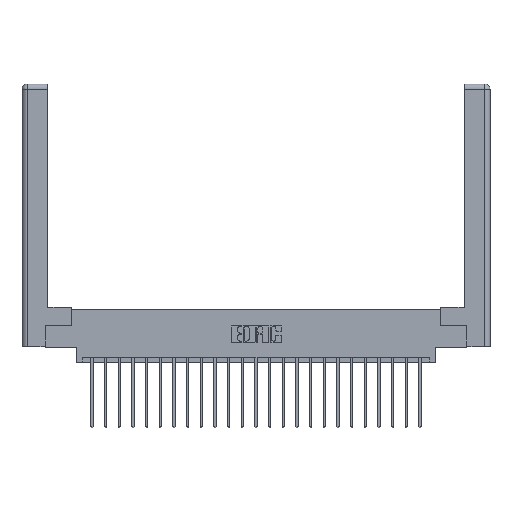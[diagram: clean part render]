
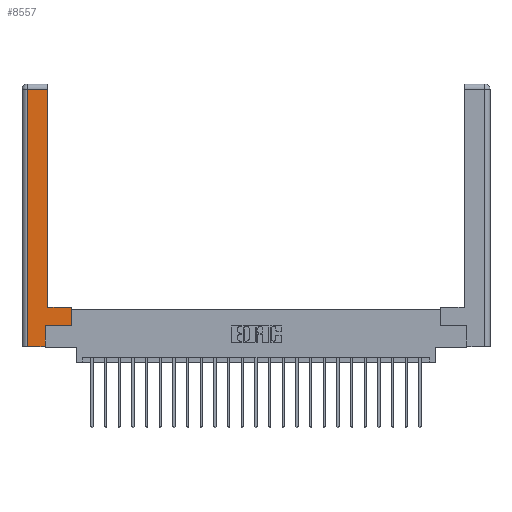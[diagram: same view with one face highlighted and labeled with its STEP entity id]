
A CAD part, top view. The second image highlights one B-rep face of the part: STEP entity #8557.
In plain terms, the highlighted planar face has unit normal (0, 0, 1).
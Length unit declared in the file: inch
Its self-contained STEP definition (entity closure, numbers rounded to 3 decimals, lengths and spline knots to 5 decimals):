
#236 = VERTEX_POINT ( 'NONE', #16291 ) ;
#309 = DIRECTION ( 'NONE',  ( -1., 0., 0. ) ) ;
#493 = LINE ( 'NONE', #4490, #4329 ) ;
#516 = CARTESIAN_POINT ( 'NONE',  ( 0.295, 2.94, 0. ) ) ;
#560 = VERTEX_POINT ( 'NONE', #11303 ) ;
#584 = LINE ( 'NONE', #3788, #7951 ) ;
#1024 = ORIENTED_EDGE ( 'NONE', *, *, #7927, .T. ) ;
#1229 = EDGE_CURVE ( 'NONE', #236, #560, #584, .T. ) ;
#1248 = EDGE_CURVE ( 'NONE', #13226, #10148, #17660, .T. ) ;
#2420 = CARTESIAN_POINT ( 'NONE',  ( 0.295, 3., 0. ) ) ;
#3190 = CARTESIAN_POINT ( 'NONE',  ( 0.295, 0.45, 0. ) ) ;
#3208 = DIRECTION ( 'NONE',  ( 0., 1., 0. ) ) ;
#3457 = EDGE_CURVE ( 'NONE', #4416, #13226, #493, .T. ) ;
#3673 = EDGE_CURVE ( 'NONE', #13757, #4416, #9888, .T. ) ;
#3763 = CARTESIAN_POINT ( 'NONE',  ( 0.265, 0., 0. ) ) ;
#3788 = CARTESIAN_POINT ( 'NONE',  ( 0.565, 0.245, 0. ) ) ;
#4329 = VECTOR ( 'NONE', #8517, 39.37008 ) ;
#4416 = VERTEX_POINT ( 'NONE', #516 ) ;
#4490 = CARTESIAN_POINT ( 'NONE',  ( 0.0615, 2.94, 0. ) ) ;
#5442 = CARTESIAN_POINT ( 'NONE',  ( 0.0615, 0., 0. ) ) ;
#6892 = DIRECTION ( 'NONE',  ( 0., 0., -1. ) ) ;
#6925 = CARTESIAN_POINT ( 'NONE',  ( 0.265, 0.245, 0. ) ) ;
#7927 = EDGE_CURVE ( 'NONE', #560, #14397, #12509, .T. ) ;
#7951 = VECTOR ( 'NONE', #22508, 39.37008 ) ;
#8245 = EDGE_CURVE ( 'NONE', #13904, #236, #17812, .T. ) ;
#8517 = DIRECTION ( 'NONE',  ( -1., 0., 0. ) ) ;
#8557 = ADVANCED_FACE ( 'NONE', ( #15566 ), #8765, .F. ) ;
#8765 = PLANE ( 'NONE',  #18455 ) ;
#9130 = ORIENTED_EDGE ( 'NONE', *, *, #23506, .T. ) ;
#9276 = VECTOR ( 'NONE', #3208, 39.37008 ) ;
#9432 = ORIENTED_EDGE ( 'NONE', *, *, #8245, .T. ) ;
#9701 = CARTESIAN_POINT ( 'NONE',  ( 0.0615, 0., 0. ) ) ;
#9888 = LINE ( 'NONE', #2420, #10201 ) ;
#10148 = VERTEX_POINT ( 'NONE', #9701 ) ;
#10201 = VECTOR ( 'NONE', #21325, 39.37008 ) ;
#10463 = VECTOR ( 'NONE', #16223, 39.37008 ) ;
#10732 = EDGE_LOOP ( 'NONE', ( #18610, #23179, #24391, #9130, #9432, #20119, #1024, #12828 ) ) ;
#11079 = CARTESIAN_POINT ( 'NONE',  ( 0.295, 0.45, 0. ) ) ;
#11303 = CARTESIAN_POINT ( 'NONE',  ( 0.565, 0.245, 0. ) ) ;
#12509 = LINE ( 'NONE', #14223, #9276 ) ;
#12828 = ORIENTED_EDGE ( 'NONE', *, *, #13923, .T. ) ;
#13226 = VERTEX_POINT ( 'NONE', #19038 ) ;
#13520 = VECTOR ( 'NONE', #16954, 39.37008 ) ;
#13757 = VERTEX_POINT ( 'NONE', #3190 ) ;
#13904 = VERTEX_POINT ( 'NONE', #3763 ) ;
#13923 = EDGE_CURVE ( 'NONE', #14397, #13757, #15468, .T. ) ;
#14094 = DIRECTION ( 'NONE',  ( -1., 0., 0. ) ) ;
#14223 = CARTESIAN_POINT ( 'NONE',  ( 0.565, 0.45, 0. ) ) ;
#14225 = VECTOR ( 'NONE', #23507, 39.37008 ) ;
#14397 = VERTEX_POINT ( 'NONE', #17704 ) ;
#15468 = LINE ( 'NONE', #11079, #23173 ) ;
#15566 = FACE_OUTER_BOUND ( 'NONE', #10732, .T. ) ;
#15822 = CARTESIAN_POINT ( 'NONE',  ( 0.265, 0., 0. ) ) ;
#16223 = DIRECTION ( 'NONE',  ( 0., 1., 0. ) ) ;
#16291 = CARTESIAN_POINT ( 'NONE',  ( 0.265, 0.245, 0. ) ) ;
#16954 = DIRECTION ( 'NONE',  ( 0., -1., 0. ) ) ;
#17660 = LINE ( 'NONE', #5442, #13520 ) ;
#17704 = CARTESIAN_POINT ( 'NONE',  ( 0.565, 0.45, 0. ) ) ;
#17812 = LINE ( 'NONE', #6925, #10463 ) ;
#18161 = CARTESIAN_POINT ( 'NONE',  ( 0., 0., 0. ) ) ;
#18455 = AXIS2_PLACEMENT_3D ( 'NONE', #18161, #6892, #14094 ) ;
#18610 = ORIENTED_EDGE ( 'NONE', *, *, #3673, .T. ) ;
#18649 = LINE ( 'NONE', #15822, #14225 ) ;
#19038 = CARTESIAN_POINT ( 'NONE',  ( 0.0615, 2.94, 0. ) ) ;
#20119 = ORIENTED_EDGE ( 'NONE', *, *, #1229, .T. ) ;
#21325 = DIRECTION ( 'NONE',  ( 0., 1., 0. ) ) ;
#22508 = DIRECTION ( 'NONE',  ( 1., 0., 0. ) ) ;
#23173 = VECTOR ( 'NONE', #309, 39.37008 ) ;
#23179 = ORIENTED_EDGE ( 'NONE', *, *, #3457, .T. ) ;
#23506 = EDGE_CURVE ( 'NONE', #10148, #13904, #18649, .T. ) ;
#23507 = DIRECTION ( 'NONE',  ( 1., 0., 0. ) ) ;
#24391 = ORIENTED_EDGE ( 'NONE', *, *, #1248, .T. ) ;
